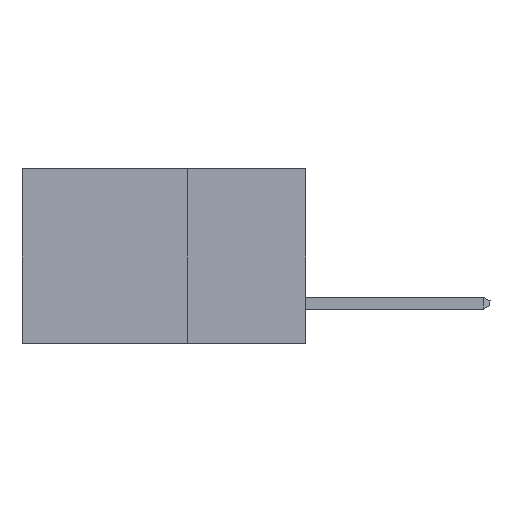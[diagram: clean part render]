
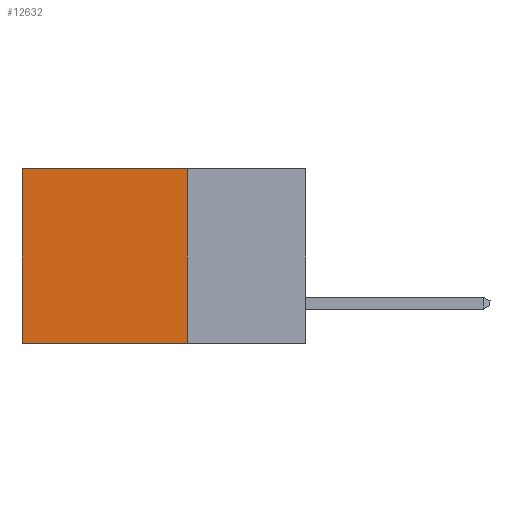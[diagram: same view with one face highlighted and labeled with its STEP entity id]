
A CAD part, left-side view. The second image highlights one B-rep face of the part: STEP entity #12632.
In plain terms, the highlighted planar face has unit normal (-1, 0, 0).
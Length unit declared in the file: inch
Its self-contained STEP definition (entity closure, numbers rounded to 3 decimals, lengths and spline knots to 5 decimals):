
#40 = EDGE_CURVE ( 'NONE', #13704, #10158, #4681, .T. ) ;
#1063 = DIRECTION ( 'NONE',  ( 1., 0., 0. ) ) ;
#1412 = VERTEX_POINT ( 'NONE', #2914 ) ;
#2274 = PLANE ( 'NONE',  #16055 ) ;
#2645 = EDGE_CURVE ( 'NONE', #1412, #10158, #11511, .T. ) ;
#2914 = CARTESIAN_POINT ( 'NONE',  ( 0.2615, 0.6, 0. ) ) ;
#3184 = CARTESIAN_POINT ( 'NONE',  ( 0.2615, 0.6, -0.37 ) ) ;
#3215 = VECTOR ( 'NONE', #10272, 39.37008 ) ;
#3510 = FACE_OUTER_BOUND ( 'NONE', #12245, .T. ) ;
#3616 = LINE ( 'NONE', #16261, #7621 ) ;
#3911 = ORIENTED_EDGE ( 'NONE', *, *, #5917, .F. ) ;
#4656 = VECTOR ( 'NONE', #7002, 39.37008 ) ;
#4681 = LINE ( 'NONE', #9730, #4656 ) ;
#4724 = ORIENTED_EDGE ( 'NONE', *, *, #13389, .T. ) ;
#4854 = DIRECTION ( 'NONE',  ( 0., 1., 0. ) ) ;
#5674 = LINE ( 'NONE', #11046, #15650 ) ;
#5917 = EDGE_CURVE ( 'NONE', #10683, #13704, #5674, .T. ) ;
#6074 = ORIENTED_EDGE ( 'NONE', *, *, #40, .F. ) ;
#6918 = DIRECTION ( 'NONE',  ( 0., 0., -1. ) ) ;
#7002 = DIRECTION ( 'NONE',  ( 0., 1., 0. ) ) ;
#7305 = CARTESIAN_POINT ( 'NONE',  ( 0.2615, 0.25, -0.37 ) ) ;
#7621 = VECTOR ( 'NONE', #4854, 39.37008 ) ;
#9033 = CARTESIAN_POINT ( 'NONE',  ( 0.2615, 0.6, -0.37 ) ) ;
#9730 = CARTESIAN_POINT ( 'NONE',  ( 0.2615, 0.25, -0.37 ) ) ;
#9995 = CARTESIAN_POINT ( 'NONE',  ( 0.2615, 0.25, 0. ) ) ;
#10158 = VERTEX_POINT ( 'NONE', #3184 ) ;
#10272 = DIRECTION ( 'NONE',  ( 0., 0., -1. ) ) ;
#10683 = VERTEX_POINT ( 'NONE', #9995 ) ;
#11046 = CARTESIAN_POINT ( 'NONE',  ( 0.2615, 0.25, -0.37 ) ) ;
#11511 = LINE ( 'NONE', #9033, #3215 ) ;
#12245 = EDGE_LOOP ( 'NONE', ( #13647, #6074, #3911, #4724 ) ) ;
#12359 = DIRECTION ( 'NONE',  ( 0., 0., -1. ) ) ;
#12632 = ADVANCED_FACE ( 'NONE', ( #3510 ), #2274, .F. ) ;
#13273 = CARTESIAN_POINT ( 'NONE',  ( 0.2615, 0.25, -0.37 ) ) ;
#13389 = EDGE_CURVE ( 'NONE', #10683, #1412, #3616, .T. ) ;
#13647 = ORIENTED_EDGE ( 'NONE', *, *, #2645, .T. ) ;
#13704 = VERTEX_POINT ( 'NONE', #13273 ) ;
#15650 = VECTOR ( 'NONE', #6918, 39.37008 ) ;
#16055 = AXIS2_PLACEMENT_3D ( 'NONE', #7305, #1063, #12359 ) ;
#16261 = CARTESIAN_POINT ( 'NONE',  ( 0.2615, 0.25, 0. ) ) ;
